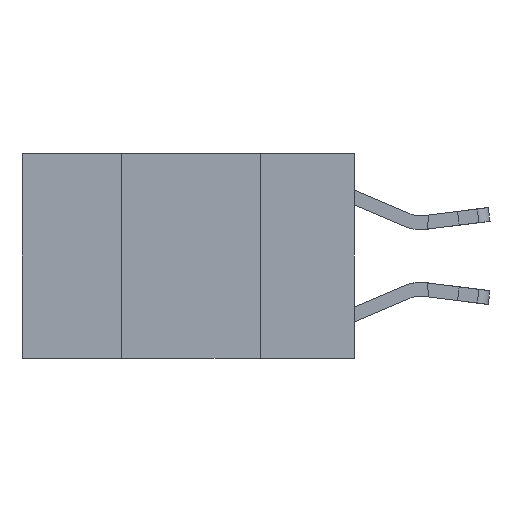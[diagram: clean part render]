
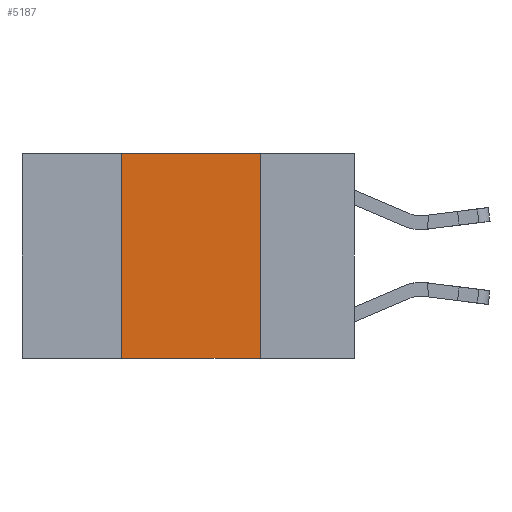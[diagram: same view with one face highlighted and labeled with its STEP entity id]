
A CAD part, left-side view. The second image highlights one B-rep face of the part: STEP entity #5187.
In plain terms, the highlighted planar face has unit normal (-1, 0, 0).
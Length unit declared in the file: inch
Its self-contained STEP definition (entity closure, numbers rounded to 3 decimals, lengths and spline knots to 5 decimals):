
#235 = CARTESIAN_POINT ( 'NONE',  ( 0., 0.42, 0. ) ) ;
#598 = ORIENTED_EDGE ( 'NONE', *, *, #2443, .F. ) ;
#619 = ORIENTED_EDGE ( 'NONE', *, *, #5742, .T. ) ;
#864 = LINE ( 'NONE', #8297, #12145 ) ;
#900 = DIRECTION ( 'NONE',  ( 0., -1., 0. ) ) ;
#1288 = PLANE ( 'NONE',  #11868 ) ;
#1963 = CARTESIAN_POINT ( 'NONE',  ( 0., 0.17, -0.37 ) ) ;
#2119 = ORIENTED_EDGE ( 'NONE', *, *, #5935, .F. ) ;
#2443 = EDGE_CURVE ( 'NONE', #14313, #9782, #3308, .T. ) ;
#2799 = ORIENTED_EDGE ( 'NONE', *, *, #6233, .F. ) ;
#2803 = LINE ( 'NONE', #4235, #8920 ) ;
#3168 = VECTOR ( 'NONE', #900, 39.37008 ) ;
#3308 = LINE ( 'NONE', #4982, #6373 ) ;
#4235 = CARTESIAN_POINT ( 'NONE',  ( 0., 0.17, 0. ) ) ;
#4889 = CARTESIAN_POINT ( 'NONE',  ( 0., 0.6, 0. ) ) ;
#4982 = CARTESIAN_POINT ( 'NONE',  ( 0., 0.42, 0. ) ) ;
#5005 = VERTEX_POINT ( 'NONE', #1963 ) ;
#5187 = ADVANCED_FACE ( 'NONE', ( #14071 ), #1288, .F. ) ;
#5742 = EDGE_CURVE ( 'NONE', #14313, #5005, #864, .T. ) ;
#5935 = EDGE_CURVE ( 'NONE', #7146, #5005, #2803, .T. ) ;
#6049 = DIRECTION ( 'NONE',  ( 1., 0., 0. ) ) ;
#6223 = LINE ( 'NONE', #14194, #3168 ) ;
#6233 = EDGE_CURVE ( 'NONE', #9782, #7146, #6223, .T. ) ;
#6255 = EDGE_LOOP ( 'NONE', ( #2119, #2799, #598, #619 ) ) ;
#6373 = VECTOR ( 'NONE', #8019, 39.37008 ) ;
#7146 = VERTEX_POINT ( 'NONE', #7942 ) ;
#7942 = CARTESIAN_POINT ( 'NONE',  ( 0., 0.17, 0. ) ) ;
#8019 = DIRECTION ( 'NONE',  ( 0., 0., 1. ) ) ;
#8297 = CARTESIAN_POINT ( 'NONE',  ( 0., 0.6, -0.37 ) ) ;
#8920 = VECTOR ( 'NONE', #9883, 39.37008 ) ;
#9376 = DIRECTION ( 'NONE',  ( 0., -1., 0. ) ) ;
#9782 = VERTEX_POINT ( 'NONE', #235 ) ;
#9883 = DIRECTION ( 'NONE',  ( 0., 0., -1. ) ) ;
#10198 = CARTESIAN_POINT ( 'NONE',  ( 0., 0.42, -0.37 ) ) ;
#11868 = AXIS2_PLACEMENT_3D ( 'NONE', #4889, #6049, #13512 ) ;
#12145 = VECTOR ( 'NONE', #9376, 39.37008 ) ;
#13512 = DIRECTION ( 'NONE',  ( 0., 0., -1. ) ) ;
#14071 = FACE_OUTER_BOUND ( 'NONE', #6255, .T. ) ;
#14194 = CARTESIAN_POINT ( 'NONE',  ( 0., 0.6, 0. ) ) ;
#14313 = VERTEX_POINT ( 'NONE', #10198 ) ;
